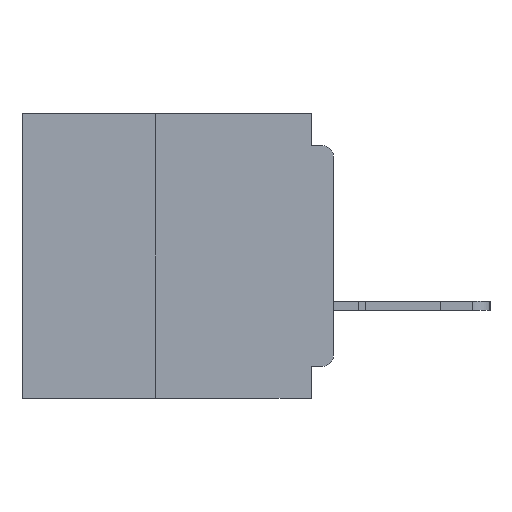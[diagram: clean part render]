
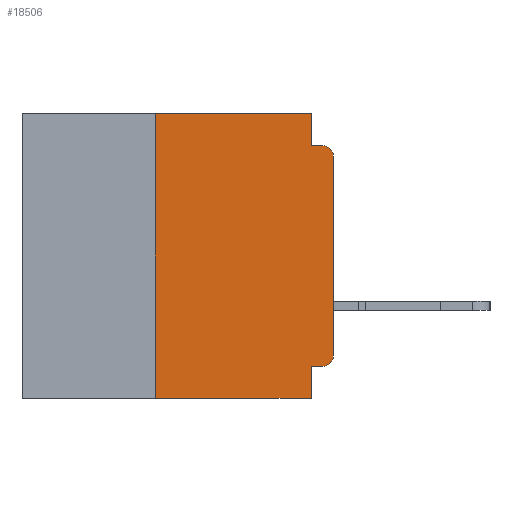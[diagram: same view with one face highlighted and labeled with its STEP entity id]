
A CAD part, left-side view. The second image highlights one B-rep face of the part: STEP entity #18506.
In plain terms, the highlighted planar face has unit normal (-1, 0, 0).
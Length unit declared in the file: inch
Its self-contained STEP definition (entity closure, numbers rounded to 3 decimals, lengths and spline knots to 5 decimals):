
#324 = VECTOR ( 'NONE', #46749, 39.37008 ) ;
#1180 = AXIS2_PLACEMENT_3D ( 'NONE', #22866, #57096, #27796 ) ;
#1628 = ORIENTED_EDGE ( 'NONE', *, *, #8728, .F. ) ;
#1856 = LINE ( 'NONE', #31991, #324 ) ;
#2298 = EDGE_CURVE ( 'NONE', #51931, #13178, #63289, .T. ) ;
#2472 = CARTESIAN_POINT ( 'NONE',  ( 0., 0.031, 0. ) ) ;
#3070 = CARTESIAN_POINT ( 'NONE',  ( 0., 0., -0.06 ) ) ;
#3620 = CARTESIAN_POINT ( 'NONE',  ( 0., 0.437, 0. ) ) ;
#3850 = DIRECTION ( 'NONE',  ( 0., 1., 0. ) ) ;
#3966 = PLANE ( 'NONE',  #5547 ) ;
#4638 = VERTEX_POINT ( 'NONE', #21039 ) ;
#4838 = VECTOR ( 'NONE', #49955, 39.37008 ) ;
#5547 = AXIS2_PLACEMENT_3D ( 'NONE', #28435, #38300, #8852 ) ;
#5862 = VERTEX_POINT ( 'NONE', #56325 ) ;
#6094 = ORIENTED_EDGE ( 'NONE', *, *, #62039, .F. ) ;
#7718 = EDGE_CURVE ( 'NONE', #5862, #20472, #1856, .T. ) ;
#7823 = FACE_OUTER_BOUND ( 'NONE', #35791, .T. ) ;
#8481 = EDGE_CURVE ( 'NONE', #4638, #62440, #34055, .T. ) ;
#8728 = EDGE_CURVE ( 'NONE', #50400, #5862, #40985, .T. ) ;
#8852 = DIRECTION ( 'NONE',  ( 0., 0., -1. ) ) ;
#9823 = LINE ( 'NONE', #3620, #21354 ) ;
#11249 = ORIENTED_EDGE ( 'NONE', *, *, #2298, .T. ) ;
#11354 = CARTESIAN_POINT ( 'NONE',  ( 0., 0.015, -0.045 ) ) ;
#11412 = ORIENTED_EDGE ( 'NONE', *, *, #7718, .F. ) ;
#12594 = ORIENTED_EDGE ( 'NONE', *, *, #8481, .F. ) ;
#12638 = VERTEX_POINT ( 'NONE', #2472 ) ;
#12898 = DIRECTION ( 'NONE',  ( 0., -1., 0. ) ) ;
#13178 = VERTEX_POINT ( 'NONE', #3070 ) ;
#14300 = EDGE_CURVE ( 'NONE', #62440, #12638, #9823, .T. ) ;
#14530 = ORIENTED_EDGE ( 'NONE', *, *, #18756, .T. ) ;
#14734 = ORIENTED_EDGE ( 'NONE', *, *, #14300, .F. ) ;
#18506 = ADVANCED_FACE ( 'NONE', ( #7823 ), #3966, .F. ) ;
#18756 = EDGE_CURVE ( 'NONE', #13178, #24946, #26615, .T. ) ;
#18788 = DIRECTION ( 'NONE',  ( 0., 0., -1. ) ) ;
#19882 = ORIENTED_EDGE ( 'NONE', *, *, #38691, .T. ) ;
#20472 = VERTEX_POINT ( 'NONE', #62619 ) ;
#20560 = VECTOR ( 'NONE', #18788, 39.37008 ) ;
#20846 = CARTESIAN_POINT ( 'NONE',  ( 0., 0.015, -0.06 ) ) ;
#21039 = CARTESIAN_POINT ( 'NONE',  ( 0., 0.25, -0.4 ) ) ;
#21354 = VECTOR ( 'NONE', #62275, 39.37008 ) ;
#22255 = VECTOR ( 'NONE', #12898, 39.37008 ) ;
#22866 = CARTESIAN_POINT ( 'NONE',  ( 0., 0.015, -0.34 ) ) ;
#23797 = LINE ( 'NONE', #42364, #22255 ) ;
#24946 = VERTEX_POINT ( 'NONE', #11354 ) ;
#25288 = EDGE_CURVE ( 'NONE', #47336, #24946, #58444, .T. ) ;
#25486 = CARTESIAN_POINT ( 'NONE',  ( 0., 0.25, -0.4 ) ) ;
#25771 = DIRECTION ( 'NONE',  ( 0., 0., -1. ) ) ;
#26615 = CIRCLE ( 'NONE', #58085, 0.015 ) ;
#27796 = DIRECTION ( 'NONE',  ( 0., 0., -1. ) ) ;
#27944 = VECTOR ( 'NONE', #3850, 39.37008 ) ;
#28435 = CARTESIAN_POINT ( 'NONE',  ( 0., 0.437, 0. ) ) ;
#31991 = CARTESIAN_POINT ( 'NONE',  ( 0., 0.031, -0.4 ) ) ;
#33682 = LINE ( 'NONE', #38355, #20560 ) ;
#33707 = EDGE_CURVE ( 'NONE', #50400, #51931, #41411, .T. ) ;
#34055 = LINE ( 'NONE', #25486, #4838 ) ;
#35210 = CARTESIAN_POINT ( 'NONE',  ( 0., 0.031, -0.045 ) ) ;
#35791 = EDGE_LOOP ( 'NONE', ( #11249, #14530, #43087, #6094, #14734, #12594, #19882, #11412, #1628, #49923 ) ) ;
#37792 = DIRECTION ( 'NONE',  ( 0., -1., 0. ) ) ;
#38300 = DIRECTION ( 'NONE',  ( 1., 0., 0. ) ) ;
#38355 = CARTESIAN_POINT ( 'NONE',  ( 0., 0.031, 0. ) ) ;
#38691 = EDGE_CURVE ( 'NONE', #4638, #20472, #23797, .T. ) ;
#40418 = DIRECTION ( 'NONE',  ( 0., 0., 1. ) ) ;
#40985 = LINE ( 'NONE', #43110, #27944 ) ;
#41411 = CIRCLE ( 'NONE', #1180, 0.015 ) ;
#42364 = CARTESIAN_POINT ( 'NONE',  ( 0., 0.437, -0.4 ) ) ;
#43087 = ORIENTED_EDGE ( 'NONE', *, *, #25288, .F. ) ;
#43110 = CARTESIAN_POINT ( 'NONE',  ( 0., 0., -0.355 ) ) ;
#46749 = DIRECTION ( 'NONE',  ( 0., 0., -1. ) ) ;
#47336 = VERTEX_POINT ( 'NONE', #35210 ) ;
#47911 = CARTESIAN_POINT ( 'NONE',  ( 0., 0., 0. ) ) ;
#49923 = ORIENTED_EDGE ( 'NONE', *, *, #33707, .T. ) ;
#49955 = DIRECTION ( 'NONE',  ( 0., 0., 1. ) ) ;
#50347 = VECTOR ( 'NONE', #40418, 39.37008 ) ;
#50400 = VERTEX_POINT ( 'NONE', #52173 ) ;
#51931 = VERTEX_POINT ( 'NONE', #59913 ) ;
#52173 = CARTESIAN_POINT ( 'NONE',  ( 0., 0.015, -0.355 ) ) ;
#55105 = DIRECTION ( 'NONE',  ( -1., 0., 0. ) ) ;
#56325 = CARTESIAN_POINT ( 'NONE',  ( 0., 0.031, -0.355 ) ) ;
#56925 = VECTOR ( 'NONE', #37792, 39.37008 ) ;
#57096 = DIRECTION ( 'NONE',  ( -1., 0., 0. ) ) ;
#57421 = CARTESIAN_POINT ( 'NONE',  ( 0., 0., -0.045 ) ) ;
#58085 = AXIS2_PLACEMENT_3D ( 'NONE', #20846, #55105, #25771 ) ;
#58444 = LINE ( 'NONE', #57421, #56925 ) ;
#59913 = CARTESIAN_POINT ( 'NONE',  ( 0., 0., -0.34 ) ) ;
#60935 = CARTESIAN_POINT ( 'NONE',  ( 0., 0.25, 0. ) ) ;
#62039 = EDGE_CURVE ( 'NONE', #12638, #47336, #33682, .T. ) ;
#62275 = DIRECTION ( 'NONE',  ( 0., -1., 0. ) ) ;
#62440 = VERTEX_POINT ( 'NONE', #60935 ) ;
#62619 = CARTESIAN_POINT ( 'NONE',  ( 0., 0.031, -0.4 ) ) ;
#63289 = LINE ( 'NONE', #47911, #50347 ) ;
